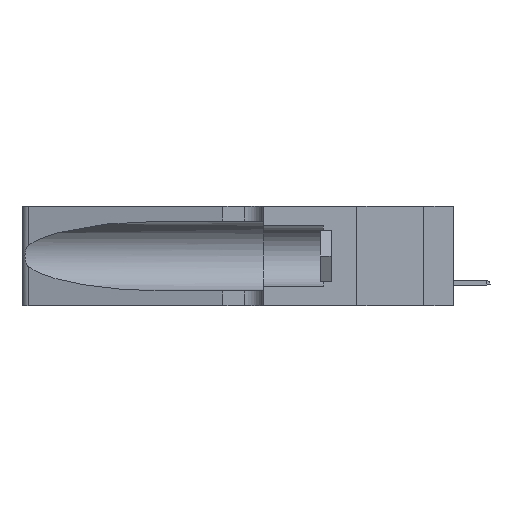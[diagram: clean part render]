
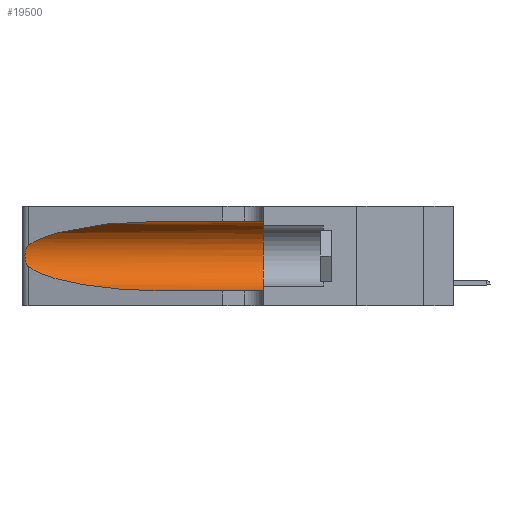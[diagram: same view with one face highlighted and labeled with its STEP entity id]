
A CAD part, left-side view. The second image highlights one B-rep face of the part: STEP entity #19500.
In plain terms, the highlighted cylindrical face has radius 3.308 mm (diameter 6.617 mm), a partial arc.
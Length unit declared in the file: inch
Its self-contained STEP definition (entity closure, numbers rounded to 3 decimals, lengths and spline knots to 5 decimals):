
#499 = CARTESIAN_POINT ( 'NONE',  ( 0.1305, 0.35, 0.05475 ) ) ;
#554 = CARTESIAN_POINT ( 'NONE',  ( 0.18966, 0.96281, 0.05475 ) ) ;
#1515 = LINE ( 'NONE', #16072, #1815 ) ;
#1622 = CARTESIAN_POINT ( 'NONE',  ( 0.1305, 0.35, 0.31525 ) ) ;
#1628 = EDGE_CURVE ( 'NONE', #6216, #5062, #19846, .T. ) ;
#1700 = CARTESIAN_POINT ( 'NONE',  ( 0.26017, 1.23833, 0.17102 ) ) ;
#1815 = VECTOR ( 'NONE', #21373, 39.37008 ) ;
#2035 = CARTESIAN_POINT ( 'NONE',  ( 0.25487, 1.22718, 0.22369 ) ) ;
#2167 = CARTESIAN_POINT ( 'NONE',  ( 0.26018, 1.23835, 0.19895 ) ) ;
#2766 = VERTEX_POINT ( 'NONE', #18873 ) ;
#2958 = ORIENTED_EDGE ( 'NONE', *, *, #7007, .T. ) ;
#3844 = ORIENTED_EDGE ( 'NONE', *, *, #1628, .F. ) ;
#3959 = CARTESIAN_POINT ( 'NONE',  ( 0.25555, 1.22994, 0.2215 ) ) ;
#4616 = VECTOR ( 'NONE', #10961, 39.37008 ) ;
#5062 = VERTEX_POINT ( 'NONE', #1622 ) ;
#5670 = ORIENTED_EDGE ( 'NONE', *, *, #15878, .T. ) ;
#5684 = CARTESIAN_POINT ( 'NONE',  ( 0.25487, 1.22718, 0.22369 ) ) ;
#6216 = VERTEX_POINT ( 'NONE', #17774 ) ;
#6238 = CARTESIAN_POINT ( 'NONE',  ( 0.1305, 0.72297, 0.05475 ) ) ;
#6245 = CYLINDRICAL_SURFACE ( 'NONE', #12241, 0.13025 ) ;
#6504 = CIRCLE ( 'NONE', #20142, 0.13025 ) ;
#7007 = EDGE_CURVE ( 'NONE', #17433, #2766, #17760, .T. ) ;
#8027 = ORIENTED_EDGE ( 'NONE', *, *, #11260, .T. ) ;
#8093 = CARTESIAN_POINT ( 'NONE',  ( 0.18966, 0.96281, 0.31525 ) ) ;
#8534 = DIRECTION ( 'NONE',  ( 0., 0., -1. ) ) ;
#8984 = CARTESIAN_POINT ( 'NONE',  ( 0.25856, 1.23593, 0.16098 ) ) ;
#9874 = DIRECTION ( 'NONE',  ( 0., 1., 0. ) ) ;
#10094 =( BOUNDED_CURVE ( )  B_SPLINE_CURVE ( 3, ( #17153, #8093, #21979, #5684 ),
 .UNSPECIFIED., .F., .T. ) 
 B_SPLINE_CURVE_WITH_KNOTS ( ( 4, 4 ),
 ( 1.5708, 2.84003 ),
 .UNSPECIFIED. ) 
 CURVE ( )  GEOMETRIC_REPRESENTATION_ITEM ( )  RATIONAL_B_SPLINE_CURVE ( ( 1., 0.87, 0.87, 1. ) ) 
 REPRESENTATION_ITEM ( '' )  );
#10197 = FACE_OUTER_BOUND ( 'NONE', #21573, .T. ) ;
#10961 = DIRECTION ( 'NONE',  ( 0., -1., 0. ) ) ;
#11137 = CARTESIAN_POINT ( 'NONE',  ( 0.26075, 1.23896, 0.19203 ) ) ;
#11248 = CARTESIAN_POINT ( 'NONE',  ( 0.25639, 1.23184, 0.21858 ) ) ;
#11260 = EDGE_CURVE ( 'NONE', #21349, #14801, #1515, .T. ) ;
#11408 = CARTESIAN_POINT ( 'NONE',  ( 0.2373, 1.15595, 0.08982 ) ) ;
#11815 = DIRECTION ( 'NONE',  ( 0., 0., 1. ) ) ;
#12241 = AXIS2_PLACEMENT_3D ( 'NONE', #17595, #23015, #8534 ) ;
#12565 =( BOUNDED_CURVE ( )  B_SPLINE_CURVE ( 3, ( #18982, #11408, #554, #6238 ),
 .UNSPECIFIED., .F., .T. ) 
 B_SPLINE_CURVE_WITH_KNOTS ( ( 4, 4 ),
 ( 3.44316, 4.71239 ),
 .UNSPECIFIED. ) 
 CURVE ( )  GEOMETRIC_REPRESENTATION_ITEM ( )  RATIONAL_B_SPLINE_CURVE ( ( 1., 0.87, 0.87, 1. ) ) 
 REPRESENTATION_ITEM ( '' )  );
#14801 = VERTEX_POINT ( 'NONE', #499 ) ;
#14869 = CARTESIAN_POINT ( 'NONE',  ( 0.1305, 1.61858, 0.31525 ) ) ;
#15083 = ORIENTED_EDGE ( 'NONE', *, *, #20095, .F. ) ;
#15878 = EDGE_CURVE ( 'NONE', #2766, #21349, #12565, .T. ) ;
#16072 = CARTESIAN_POINT ( 'NONE',  ( 0.1305, 1.61858, 0.05475 ) ) ;
#16492 = CARTESIAN_POINT ( 'NONE',  ( 0.25487, 1.22718, 0.14631 ) ) ;
#16719 = CARTESIAN_POINT ( 'NONE',  ( 0.25639, 1.23186, 0.15144 ) ) ;
#17153 = CARTESIAN_POINT ( 'NONE',  ( 0.1305, 0.72297, 0.31525 ) ) ;
#17412 = ORIENTED_EDGE ( 'NONE', *, *, #19046, .T. ) ;
#17433 = VERTEX_POINT ( 'NONE', #2035 ) ;
#17595 = CARTESIAN_POINT ( 'NONE',  ( 0.1305, 1.61858, 0.185 ) ) ;
#17760 = B_SPLINE_CURVE_WITH_KNOTS ( 'NONE', 3,
 ( #20219, #3959, #11248, #18262, #22126, #2167, #11137, #20002, #1700, #8984, #22019, #16719, #21783, #16492 ),
 .UNSPECIFIED., .F., .F.,
 ( 4, 2, 2, 2, 2, 2, 4 ),
 ( 0., 0.00027, 0.00053, 0.00107, 0.0016, 0.00187, 0.00214 ),
 .UNSPECIFIED. ) ;
#17774 = CARTESIAN_POINT ( 'NONE',  ( 0.1305, 0.72297, 0.31525 ) ) ;
#18262 = CARTESIAN_POINT ( 'NONE',  ( 0.25787, 1.23484, 0.2124 ) ) ;
#18873 = CARTESIAN_POINT ( 'NONE',  ( 0.25487, 1.22718, 0.14631 ) ) ;
#18982 = CARTESIAN_POINT ( 'NONE',  ( 0.25487, 1.22718, 0.14631 ) ) ;
#19046 = EDGE_CURVE ( 'NONE', #6216, #17433, #10094, .T. ) ;
#19153 = CARTESIAN_POINT ( 'NONE',  ( 0.1305, 0.72297, 0.05475 ) ) ;
#19500 = ADVANCED_FACE ( 'NONE', ( #10197 ), #6245, .F. ) ;
#19846 = LINE ( 'NONE', #14869, #4616 ) ;
#20002 = CARTESIAN_POINT ( 'NONE',  ( 0.26075, 1.23896, 0.178 ) ) ;
#20095 = EDGE_CURVE ( 'NONE', #5062, #14801, #6504, .T. ) ;
#20142 = AXIS2_PLACEMENT_3D ( 'NONE', #20789, #9874, #11815 ) ;
#20219 = CARTESIAN_POINT ( 'NONE',  ( 0.25487, 1.22718, 0.22369 ) ) ;
#20789 = CARTESIAN_POINT ( 'NONE',  ( 0.1305, 0.35, 0.185 ) ) ;
#21349 = VERTEX_POINT ( 'NONE', #19153 ) ;
#21373 = DIRECTION ( 'NONE',  ( 0., -1., 0. ) ) ;
#21573 = EDGE_LOOP ( 'NONE', ( #17412, #2958, #5670, #8027, #15083, #3844 ) ) ;
#21783 = CARTESIAN_POINT ( 'NONE',  ( 0.25555, 1.22993, 0.14849 ) ) ;
#21979 = CARTESIAN_POINT ( 'NONE',  ( 0.2373, 1.15595, 0.28018 ) ) ;
#22019 = CARTESIAN_POINT ( 'NONE',  ( 0.25789, 1.23486, 0.15765 ) ) ;
#22126 = CARTESIAN_POINT ( 'NONE',  ( 0.25854, 1.2359, 0.20912 ) ) ;
#23015 = DIRECTION ( 'NONE',  ( 0., -1., 0. ) ) ;
